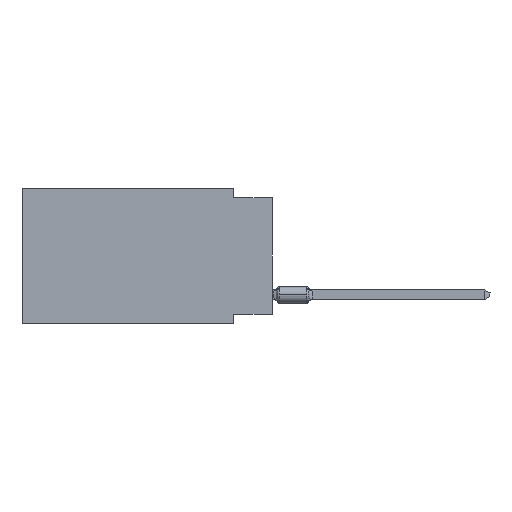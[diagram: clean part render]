
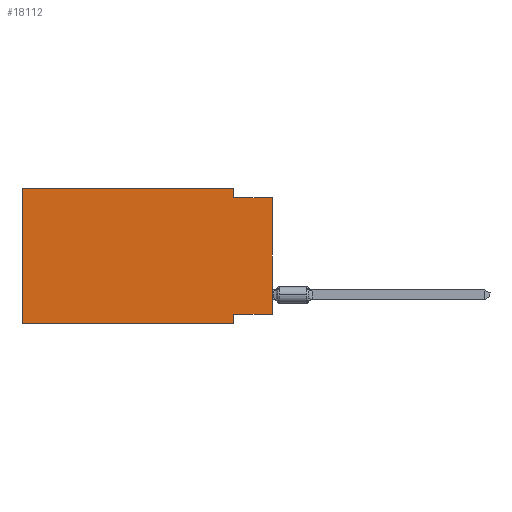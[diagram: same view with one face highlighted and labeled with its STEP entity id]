
A CAD part, left-side view. The second image highlights one B-rep face of the part: STEP entity #18112.
In plain terms, the highlighted planar face has unit normal (-1, 0, 0).
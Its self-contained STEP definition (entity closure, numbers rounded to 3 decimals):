
#935 = VERTEX_POINT ( 'NONE', #35034 ) ;
#1733 = EDGE_CURVE ( 'NONE', #75962, #67428, #9306, .T. ) ;
#3384 = LINE ( 'NONE', #72586, #27519 ) ;
#5537 = EDGE_CURVE ( 'NONE', #80552, #24208, #21438, .T. ) ;
#7133 = FACE_OUTER_BOUND ( 'NONE', #66664, .T. ) ;
#9306 = LINE ( 'NONE', #34430, #27198 ) ;
#10045 = VERTEX_POINT ( 'NONE', #30019 ) ;
#10916 = ORIENTED_EDGE ( 'NONE', *, *, #35505, .F. ) ;
#12897 = CARTESIAN_POINT ( 'NONE',  ( 0., 2.54, -0.635 ) ) ;
#14151 = LINE ( 'NONE', #63559, #81037 ) ;
#14614 = DIRECTION ( 'NONE',  ( 0., -1., 0. ) ) ;
#16982 = DIRECTION ( 'NONE',  ( 0., 0., -1. ) ) ;
#17132 = VECTOR ( 'NONE', #65048, 1000. ) ;
#18112 = ADVANCED_FACE ( 'NONE', ( #7133 ), #38438, .F. ) ;
#18217 = CARTESIAN_POINT ( 'NONE',  ( 0., 16.383, 0. ) ) ;
#18265 = VECTOR ( 'NONE', #14614, 1000. ) ;
#19934 = DIRECTION ( 'NONE',  ( 0., -1., 0. ) ) ;
#21438 = LINE ( 'NONE', #53540, #17132 ) ;
#23431 = CARTESIAN_POINT ( 'NONE',  ( 0., 2.54, 0. ) ) ;
#24208 = VERTEX_POINT ( 'NONE', #12897 ) ;
#25048 = ORIENTED_EDGE ( 'NONE', *, *, #38027, .T. ) ;
#26129 = CARTESIAN_POINT ( 'NONE',  ( 0., 0., -0.635 ) ) ;
#27198 = VECTOR ( 'NONE', #77675, 1000. ) ;
#27223 = LINE ( 'NONE', #58923, #49307 ) ;
#27519 = VECTOR ( 'NONE', #16982, 1000. ) ;
#28435 = ORIENTED_EDGE ( 'NONE', *, *, #59697, .F. ) ;
#30019 = CARTESIAN_POINT ( 'NONE',  ( 0., 16.383, 0. ) ) ;
#31042 = CARTESIAN_POINT ( 'NONE',  ( 0., 16.383, 0. ) ) ;
#33580 = EDGE_CURVE ( 'NONE', #75962, #35188, #27223, .T. ) ;
#33814 = ORIENTED_EDGE ( 'NONE', *, *, #5537, .F. ) ;
#34430 = CARTESIAN_POINT ( 'NONE',  ( 0., 0., 0. ) ) ;
#35034 = CARTESIAN_POINT ( 'NONE',  ( 0., 2.54, -8.89 ) ) ;
#35188 = VERTEX_POINT ( 'NONE', #57807 ) ;
#35505 = EDGE_CURVE ( 'NONE', #63691, #10045, #62664, .T. ) ;
#38027 = EDGE_CURVE ( 'NONE', #63691, #935, #52079, .T. ) ;
#38438 = PLANE ( 'NONE',  #53565 ) ;
#40042 = DIRECTION ( 'NONE',  ( 0., -1., 0. ) ) ;
#44177 = ORIENTED_EDGE ( 'NONE', *, *, #1733, .T. ) ;
#44313 = LINE ( 'NONE', #77536, #57124 ) ;
#45747 = ORIENTED_EDGE ( 'NONE', *, *, #33580, .F. ) ;
#49307 = VECTOR ( 'NONE', #52335, 1000. ) ;
#52079 = LINE ( 'NONE', #77216, #18265 ) ;
#52335 = DIRECTION ( 'NONE',  ( 0., 1., 0. ) ) ;
#53540 = CARTESIAN_POINT ( 'NONE',  ( 0., 2.54, 0. ) ) ;
#53565 = AXIS2_PLACEMENT_3D ( 'NONE', #31042, #69330, #68511 ) ;
#57124 = VECTOR ( 'NONE', #40042, 1000. ) ;
#57807 = CARTESIAN_POINT ( 'NONE',  ( 0., 2.54, -8.255 ) ) ;
#58747 = VECTOR ( 'NONE', #68837, 1000. ) ;
#58923 = CARTESIAN_POINT ( 'NONE',  ( 0., 0., -8.255 ) ) ;
#59697 = EDGE_CURVE ( 'NONE', #24208, #67428, #44313, .T. ) ;
#62067 = CARTESIAN_POINT ( 'NONE',  ( 0., 0., -8.255 ) ) ;
#62664 = LINE ( 'NONE', #18217, #58747 ) ;
#63559 = CARTESIAN_POINT ( 'NONE',  ( 0., 16.383, 0. ) ) ;
#63691 = VERTEX_POINT ( 'NONE', #67614 ) ;
#65048 = DIRECTION ( 'NONE',  ( 0., 0., -1. ) ) ;
#66664 = EDGE_LOOP ( 'NONE', ( #44177, #28435, #33814, #80929, #10916, #25048, #74280, #45747 ) ) ;
#67428 = VERTEX_POINT ( 'NONE', #26129 ) ;
#67614 = CARTESIAN_POINT ( 'NONE',  ( 0., 16.383, -8.89 ) ) ;
#68511 = DIRECTION ( 'NONE',  ( 0., 0., -1. ) ) ;
#68837 = DIRECTION ( 'NONE',  ( 0., 0., 1. ) ) ;
#69330 = DIRECTION ( 'NONE',  ( 1., 0., 0. ) ) ;
#72586 = CARTESIAN_POINT ( 'NONE',  ( 0., 2.54, -8.89 ) ) ;
#73648 = EDGE_CURVE ( 'NONE', #10045, #80552, #14151, .T. ) ;
#74280 = ORIENTED_EDGE ( 'NONE', *, *, #77280, .F. ) ;
#75962 = VERTEX_POINT ( 'NONE', #62067 ) ;
#77216 = CARTESIAN_POINT ( 'NONE',  ( 0., 16.383, -8.89 ) ) ;
#77280 = EDGE_CURVE ( 'NONE', #35188, #935, #3384, .T. ) ;
#77536 = CARTESIAN_POINT ( 'NONE',  ( 0., 0., -0.635 ) ) ;
#77675 = DIRECTION ( 'NONE',  ( 0., 0., 1. ) ) ;
#80552 = VERTEX_POINT ( 'NONE', #23431 ) ;
#80929 = ORIENTED_EDGE ( 'NONE', *, *, #73648, .F. ) ;
#81037 = VECTOR ( 'NONE', #19934, 1000. ) ;
